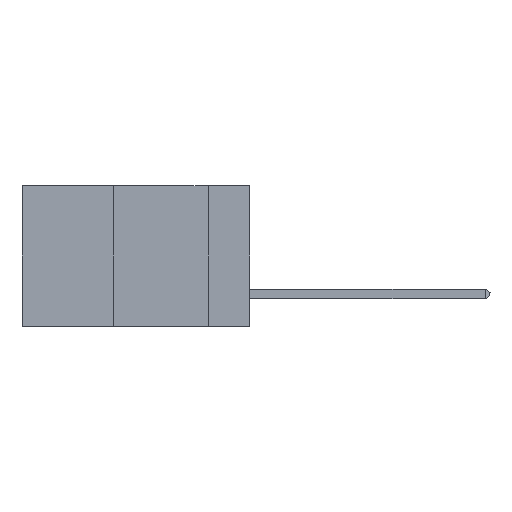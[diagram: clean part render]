
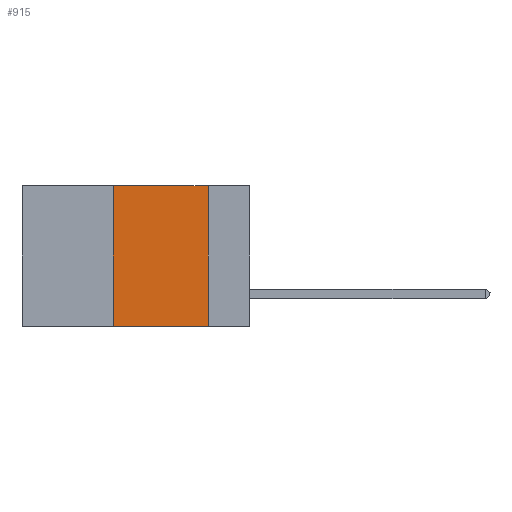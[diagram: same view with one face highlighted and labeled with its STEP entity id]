
A CAD part, left-side view. The second image highlights one B-rep face of the part: STEP entity #915.
In plain terms, the highlighted planar face has unit normal (-1, 0, 0).
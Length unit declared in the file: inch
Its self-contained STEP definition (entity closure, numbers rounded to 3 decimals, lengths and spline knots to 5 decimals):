
#627 = EDGE_LOOP ( 'NONE', ( #2419, #17719, #16560, #19382 ) ) ;
#915 = ADVANCED_FACE ( 'NONE', ( #20051 ), #2837, .F. ) ;
#1620 = CARTESIAN_POINT ( 'NONE',  ( 0., 0.11, 0. ) ) ;
#1765 = AXIS2_PLACEMENT_3D ( 'NONE', #37061, #14918, #39071 ) ;
#1945 = VERTEX_POINT ( 'NONE', #26384 ) ;
#2419 = ORIENTED_EDGE ( 'NONE', *, *, #27095, .F. ) ;
#2837 = PLANE ( 'NONE',  #1765 ) ;
#3734 = DIRECTION ( 'NONE',  ( 0., 0., 1. ) ) ;
#4075 = LINE ( 'NONE', #37669, #17358 ) ;
#4891 = LINE ( 'NONE', #29077, #27678 ) ;
#6876 = EDGE_CURVE ( 'NONE', #34320, #1945, #4891, .T. ) ;
#7905 = DIRECTION ( 'NONE',  ( 0., -1., 0. ) ) ;
#8481 = VERTEX_POINT ( 'NONE', #1620 ) ;
#10451 = VERTEX_POINT ( 'NONE', #15340 ) ;
#13274 = CARTESIAN_POINT ( 'NONE',  ( 0., 0.36, 0. ) ) ;
#14568 = VECTOR ( 'NONE', #3734, 39.37008 ) ;
#14918 = DIRECTION ( 'NONE',  ( 1., 0., 0. ) ) ;
#14931 = DIRECTION ( 'NONE',  ( 0., 0., -1. ) ) ;
#15340 = CARTESIAN_POINT ( 'NONE',  ( 0., 0.36, 0. ) ) ;
#16560 = ORIENTED_EDGE ( 'NONE', *, *, #20476, .F. ) ;
#17358 = VECTOR ( 'NONE', #19241, 39.37008 ) ;
#17592 = CARTESIAN_POINT ( 'NONE',  ( 0., 0.11, 0. ) ) ;
#17719 = ORIENTED_EDGE ( 'NONE', *, *, #23710, .F. ) ;
#19241 = DIRECTION ( 'NONE',  ( 0., -1., 0. ) ) ;
#19382 = ORIENTED_EDGE ( 'NONE', *, *, #6876, .T. ) ;
#20051 = FACE_OUTER_BOUND ( 'NONE', #627, .T. ) ;
#20476 = EDGE_CURVE ( 'NONE', #34320, #10451, #26884, .T. ) ;
#22708 = VECTOR ( 'NONE', #14931, 39.37008 ) ;
#23710 = EDGE_CURVE ( 'NONE', #10451, #8481, #4075, .T. ) ;
#26384 = CARTESIAN_POINT ( 'NONE',  ( 0., 0.11, -0.37 ) ) ;
#26884 = LINE ( 'NONE', #13274, #14568 ) ;
#27095 = EDGE_CURVE ( 'NONE', #8481, #1945, #29787, .T. ) ;
#27678 = VECTOR ( 'NONE', #7905, 39.37008 ) ;
#29077 = CARTESIAN_POINT ( 'NONE',  ( 0., 0.6, -0.37 ) ) ;
#29787 = LINE ( 'NONE', #17592, #22708 ) ;
#33843 = CARTESIAN_POINT ( 'NONE',  ( 0., 0.36, -0.37 ) ) ;
#34320 = VERTEX_POINT ( 'NONE', #33843 ) ;
#37061 = CARTESIAN_POINT ( 'NONE',  ( 0., 0.6, 0. ) ) ;
#37669 = CARTESIAN_POINT ( 'NONE',  ( 0., 0.6, 0. ) ) ;
#39071 = DIRECTION ( 'NONE',  ( 0., 0., -1. ) ) ;
